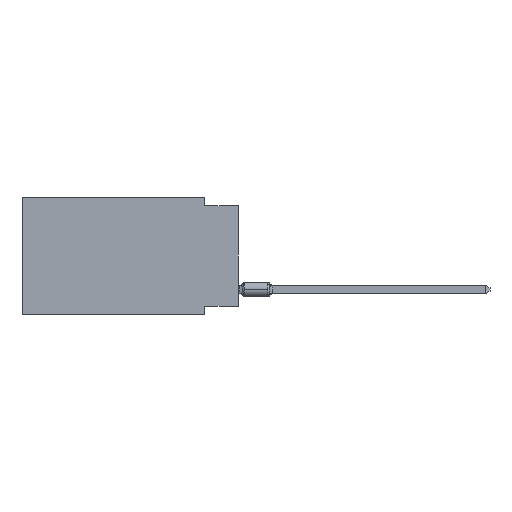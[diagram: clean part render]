
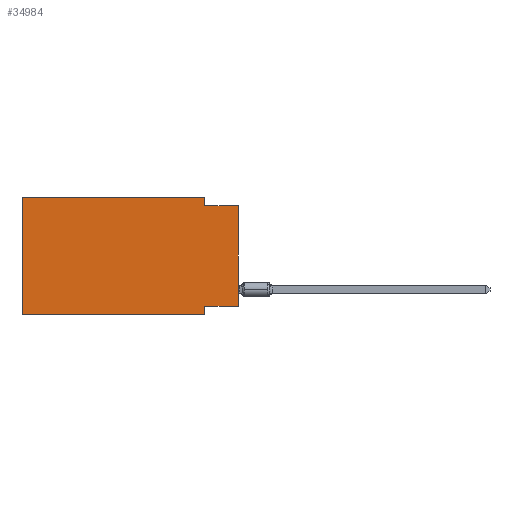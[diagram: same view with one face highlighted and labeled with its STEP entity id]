
A CAD part, left-side view. The second image highlights one B-rep face of the part: STEP entity #34984.
In plain terms, the highlighted planar face has unit normal (-1, 0, 0).
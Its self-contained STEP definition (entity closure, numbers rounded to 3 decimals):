
#715 = EDGE_CURVE ( 'NONE', #32921, #4014, #17742, .T. ) ;
#1649 = CARTESIAN_POINT ( 'NONE',  ( 0., 0., -0.635 ) ) ;
#1737 = EDGE_CURVE ( 'NONE', #20379, #35472, #27286, .T. ) ;
#2026 = CARTESIAN_POINT ( 'NONE',  ( 0., 2.54, -0.635 ) ) ;
#2141 = DIRECTION ( 'NONE',  ( 0., 0., 1. ) ) ;
#2249 = LINE ( 'NONE', #4510, #12634 ) ;
#2258 = EDGE_CURVE ( 'NONE', #31779, #14564, #9379, .T. ) ;
#4014 = VERTEX_POINT ( 'NONE', #1649 ) ;
#4149 = EDGE_CURVE ( 'NONE', #32921, #20379, #20941, .T. ) ;
#4510 = CARTESIAN_POINT ( 'NONE',  ( 0., 16.383, 0. ) ) ;
#5621 = CARTESIAN_POINT ( 'NONE',  ( 0., 0., 0. ) ) ;
#6084 = CARTESIAN_POINT ( 'NONE',  ( 0., 2.54, 0. ) ) ;
#7415 = PLANE ( 'NONE',  #17713 ) ;
#9168 = VERTEX_POINT ( 'NONE', #22696 ) ;
#9226 = CARTESIAN_POINT ( 'NONE',  ( 0., 16.383, 0. ) ) ;
#9379 = LINE ( 'NONE', #6084, #40370 ) ;
#9947 = LINE ( 'NONE', #26541, #24996 ) ;
#9985 = EDGE_LOOP ( 'NONE', ( #11540, #17617, #14083, #38001, #13478, #39410, #36031, #12914 ) ) ;
#10704 = DIRECTION ( 'NONE',  ( 1., 0., 0. ) ) ;
#11540 = ORIENTED_EDGE ( 'NONE', *, *, #715, .T. ) ;
#11839 = VECTOR ( 'NONE', #27278, 1000. ) ;
#12248 = EDGE_CURVE ( 'NONE', #22132, #35472, #33433, .T. ) ;
#12634 = VECTOR ( 'NONE', #39605, 1000. ) ;
#12857 = DIRECTION ( 'NONE',  ( 0., 0., -1. ) ) ;
#12914 = ORIENTED_EDGE ( 'NONE', *, *, #4149, .F. ) ;
#13478 = ORIENTED_EDGE ( 'NONE', *, *, #31311, .F. ) ;
#14083 = ORIENTED_EDGE ( 'NONE', *, *, #2258, .F. ) ;
#14382 = DIRECTION ( 'NONE',  ( 0., 0., -1. ) ) ;
#14564 = VERTEX_POINT ( 'NONE', #2026 ) ;
#14664 = VECTOR ( 'NONE', #2141, 1000. ) ;
#14771 = CARTESIAN_POINT ( 'NONE',  ( 0., 16.383, -8.89 ) ) ;
#16289 = DIRECTION ( 'NONE',  ( 0., -1., 0. ) ) ;
#16837 = CARTESIAN_POINT ( 'NONE',  ( 0., 16.383, 0. ) ) ;
#17617 = ORIENTED_EDGE ( 'NONE', *, *, #30191, .F. ) ;
#17713 = AXIS2_PLACEMENT_3D ( 'NONE', #16837, #10704, #14382 ) ;
#17742 = LINE ( 'NONE', #5621, #14664 ) ;
#20379 = VERTEX_POINT ( 'NONE', #23831 ) ;
#20731 = CARTESIAN_POINT ( 'NONE',  ( 0., 0., -8.255 ) ) ;
#20941 = LINE ( 'NONE', #20731, #22740 ) ;
#21528 = CARTESIAN_POINT ( 'NONE',  ( 0., 2.54, -8.89 ) ) ;
#22132 = VERTEX_POINT ( 'NONE', #36698 ) ;
#22696 = CARTESIAN_POINT ( 'NONE',  ( 0., 16.383, 0. ) ) ;
#22740 = VECTOR ( 'NONE', #33250, 1000. ) ;
#23831 = CARTESIAN_POINT ( 'NONE',  ( 0., 2.54, -8.255 ) ) ;
#24841 = CARTESIAN_POINT ( 'NONE',  ( 0., 2.54, -8.89 ) ) ;
#24996 = VECTOR ( 'NONE', #16289, 1000. ) ;
#26124 = CARTESIAN_POINT ( 'NONE',  ( 0., 2.54, 0. ) ) ;
#26459 = VECTOR ( 'NONE', #34248, 1000. ) ;
#26541 = CARTESIAN_POINT ( 'NONE',  ( 0., 0., -0.635 ) ) ;
#27278 = DIRECTION ( 'NONE',  ( 0., -1., 0. ) ) ;
#27286 = LINE ( 'NONE', #21528, #30530 ) ;
#30191 = EDGE_CURVE ( 'NONE', #14564, #4014, #9947, .T. ) ;
#30530 = VECTOR ( 'NONE', #34253, 1000. ) ;
#31147 = LINE ( 'NONE', #9226, #26459 ) ;
#31311 = EDGE_CURVE ( 'NONE', #22132, #9168, #2249, .T. ) ;
#31779 = VERTEX_POINT ( 'NONE', #26124 ) ;
#32089 = CARTESIAN_POINT ( 'NONE',  ( 0., 0., -8.255 ) ) ;
#32921 = VERTEX_POINT ( 'NONE', #32089 ) ;
#33250 = DIRECTION ( 'NONE',  ( 0., 1., 0. ) ) ;
#33433 = LINE ( 'NONE', #14771, #11839 ) ;
#33980 = EDGE_CURVE ( 'NONE', #9168, #31779, #31147, .T. ) ;
#34248 = DIRECTION ( 'NONE',  ( 0., -1., 0. ) ) ;
#34253 = DIRECTION ( 'NONE',  ( 0., 0., -1. ) ) ;
#34984 = ADVANCED_FACE ( 'NONE', ( #35532 ), #7415, .F. ) ;
#35472 = VERTEX_POINT ( 'NONE', #24841 ) ;
#35532 = FACE_OUTER_BOUND ( 'NONE', #9985, .T. ) ;
#36031 = ORIENTED_EDGE ( 'NONE', *, *, #1737, .F. ) ;
#36698 = CARTESIAN_POINT ( 'NONE',  ( 0., 16.383, -8.89 ) ) ;
#38001 = ORIENTED_EDGE ( 'NONE', *, *, #33980, .F. ) ;
#39410 = ORIENTED_EDGE ( 'NONE', *, *, #12248, .T. ) ;
#39605 = DIRECTION ( 'NONE',  ( 0., 0., 1. ) ) ;
#40370 = VECTOR ( 'NONE', #12857, 1000. ) ;
